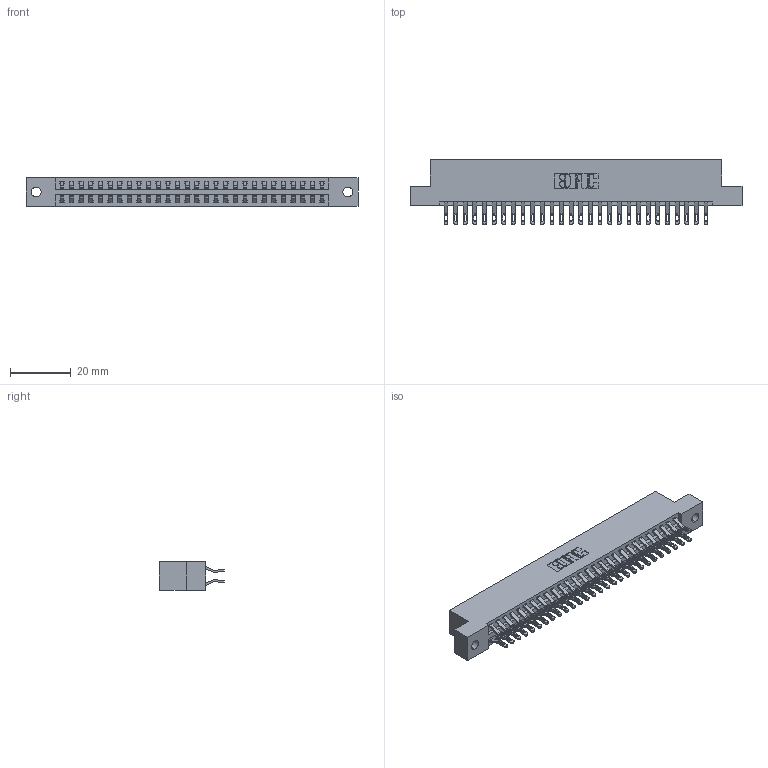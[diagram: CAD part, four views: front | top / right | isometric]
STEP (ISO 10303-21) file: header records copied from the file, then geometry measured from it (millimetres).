
FILE_DESCRIPTION (( 'STEP AP203' ), '1' );
FILE_NAME ('396-056-555-202.STEP', '2018-09-08T09:58:11', ( '' ), ( '' ), 'SwSTEP 2.0', 'SolidWorks 2016', '' );
FILE_SCHEMA (( 'CONFIG_CONTROL_DESIGN' ));
Length unit declared in the file: inch
Products named in the file (3): 396-056-555-202; 346 Part_Flush Mounting Lugs - 0.128 Dia; 345-292-001_555 Tail
Assembly tree (57 placements, depth 2):
  396-056-555-202
    346 Part_Flush Mounting Lugs - 0.128 Dia
    345-292-001_555 Tail  x56
Bounding box: 109.47 x 21.46 x 9.4 mm (x, y, z)
Volume: 10692.1 mm3; surface area: 14786.7 mm2
Topology: 57 solids, 57 shells, 3370 faces, 10577 edges, 7050 vertices
Faces by surface type: plane 1924, cylinder 1446
Entity records: 20487 total; most frequent: CARTESIAN_POINT 3430, ORIENTED_EDGE 3334, DIRECTION 3043, EDGE_CURVE 1667, LINE 1403, VECTOR 1403, VERTEX_POINT 1110, AXIS2_PLACEMENT_3D 820
